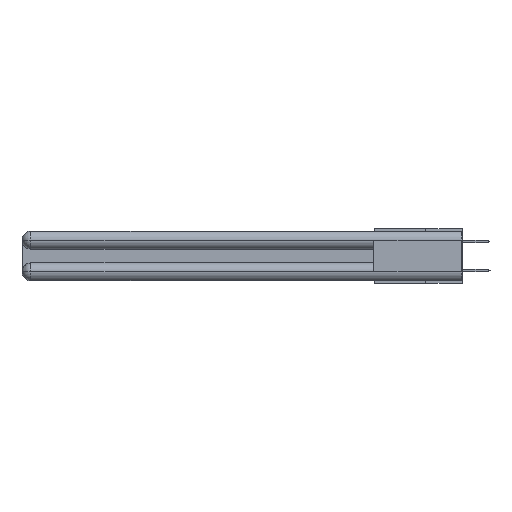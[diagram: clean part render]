
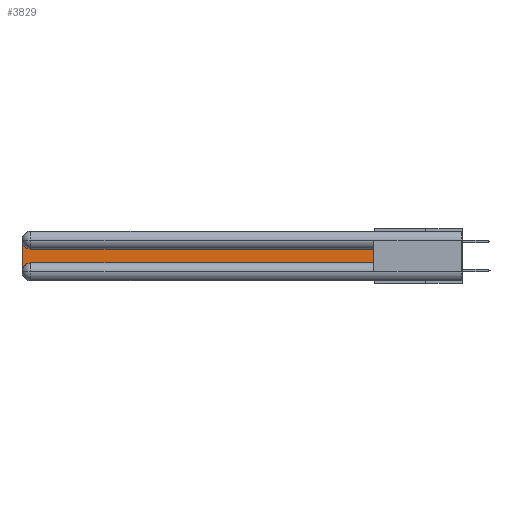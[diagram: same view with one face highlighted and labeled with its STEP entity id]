
A CAD part, left-side view. The second image highlights one B-rep face of the part: STEP entity #3829.
In plain terms, the highlighted planar face has unit normal (-1, 0, 0).
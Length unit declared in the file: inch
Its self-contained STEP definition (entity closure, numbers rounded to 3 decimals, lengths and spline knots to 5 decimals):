
#58 = DIRECTION ( 'NONE',  ( 0., 0., 1. ) ) ;
#1178 = CIRCLE ( 'NONE', #17197, 0.06 ) ;
#1445 = VECTOR ( 'NONE', #58, 39.37008 ) ;
#2576 = VECTOR ( 'NONE', #8021, 39.37008 ) ;
#2670 = CARTESIAN_POINT ( 'NONE',  ( 0.075, 3., -0.0625 ) ) ;
#2958 = PLANE ( 'NONE',  #8251 ) ;
#3028 = EDGE_CURVE ( 'NONE', #10131, #6371, #24535, .T. ) ;
#3141 = DIRECTION ( 'NONE',  ( 1., 0., 0. ) ) ;
#3829 = ADVANCED_FACE ( 'NONE', ( #7758 ), #2958, .F. ) ;
#3873 = CARTESIAN_POINT ( 'NONE',  ( 0.075, 0.6, -0.2175 ) ) ;
#4285 = DIRECTION ( 'NONE',  ( 0., 1., 0. ) ) ;
#4865 = EDGE_CURVE ( 'NONE', #14821, #15504, #6670, .T. ) ;
#5392 = ORIENTED_EDGE ( 'NONE', *, *, #4865, .T. ) ;
#5545 = ORIENTED_EDGE ( 'NONE', *, *, #15381, .T. ) ;
#6146 = CARTESIAN_POINT ( 'NONE',  ( 0.075, 2.94, -0.0625 ) ) ;
#6371 = VERTEX_POINT ( 'NONE', #9166 ) ;
#6670 = LINE ( 'NONE', #3873, #2576 ) ;
#7074 = EDGE_CURVE ( 'NONE', #27422, #10131, #8944, .T. ) ;
#7758 = FACE_OUTER_BOUND ( 'NONE', #18519, .T. ) ;
#7815 = VECTOR ( 'NONE', #28154, 39.37008 ) ;
#7866 = CARTESIAN_POINT ( 'NONE',  ( 0.075, 0.6, -0.2175 ) ) ;
#7909 = EDGE_CURVE ( 'NONE', #27952, #27422, #17935, .T. ) ;
#8021 = DIRECTION ( 'NONE',  ( 0., -1., 0. ) ) ;
#8251 = AXIS2_PLACEMENT_3D ( 'NONE', #16170, #3141, #18395 ) ;
#8944 = CIRCLE ( 'NONE', #21641, 0.06 ) ;
#9101 = CARTESIAN_POINT ( 'NONE',  ( 0.075, 2.94, -0.2775 ) ) ;
#9166 = CARTESIAN_POINT ( 'NONE',  ( 0.075, 3., -0.2775 ) ) ;
#10131 = VERTEX_POINT ( 'NONE', #2670 ) ;
#10805 = CARTESIAN_POINT ( 'NONE',  ( 0.075, 0.6, -0.2175 ) ) ;
#11217 = EDGE_CURVE ( 'NONE', #15504, #27952, #22211, .T. ) ;
#12655 = CARTESIAN_POINT ( 'NONE',  ( 0.075, 2.94, -0.2175 ) ) ;
#14821 = VERTEX_POINT ( 'NONE', #12655 ) ;
#15381 = EDGE_CURVE ( 'NONE', #6371, #14821, #1178, .T. ) ;
#15504 = VERTEX_POINT ( 'NONE', #7866 ) ;
#15704 = ORIENTED_EDGE ( 'NONE', *, *, #3028, .T. ) ;
#16170 = CARTESIAN_POINT ( 'NONE',  ( 0.075, 3., -0.1225 ) ) ;
#17197 = AXIS2_PLACEMENT_3D ( 'NONE', #9101, #25981, #24381 ) ;
#17312 = CARTESIAN_POINT ( 'NONE',  ( 0.075, 0.6, -0.1225 ) ) ;
#17377 = CARTESIAN_POINT ( 'NONE',  ( 0.075, 3., -0.2175 ) ) ;
#17935 = LINE ( 'NONE', #17312, #23753 ) ;
#18395 = DIRECTION ( 'NONE',  ( 0., 0., -1. ) ) ;
#18519 = EDGE_LOOP ( 'NONE', ( #23329, #25066, #15704, #5545, #5392, #22418 ) ) ;
#21641 = AXIS2_PLACEMENT_3D ( 'NONE', #6146, #21686, #23689 ) ;
#21686 = DIRECTION ( 'NONE',  ( 1., 0., 0. ) ) ;
#22211 = LINE ( 'NONE', #10805, #1445 ) ;
#22418 = ORIENTED_EDGE ( 'NONE', *, *, #11217, .T. ) ;
#23329 = ORIENTED_EDGE ( 'NONE', *, *, #7909, .T. ) ;
#23689 = DIRECTION ( 'NONE',  ( 0., 0., -1. ) ) ;
#23753 = VECTOR ( 'NONE', #4285, 39.37008 ) ;
#24381 = DIRECTION ( 'NONE',  ( 0., 0., -1. ) ) ;
#24535 = LINE ( 'NONE', #17377, #7815 ) ;
#25066 = ORIENTED_EDGE ( 'NONE', *, *, #7074, .T. ) ;
#25699 = CARTESIAN_POINT ( 'NONE',  ( 0.075, 2.94, -0.1225 ) ) ;
#25936 = CARTESIAN_POINT ( 'NONE',  ( 0.075, 0.6, -0.1225 ) ) ;
#25981 = DIRECTION ( 'NONE',  ( 1., 0., 0. ) ) ;
#27422 = VERTEX_POINT ( 'NONE', #25699 ) ;
#27952 = VERTEX_POINT ( 'NONE', #25936 ) ;
#28154 = DIRECTION ( 'NONE',  ( 0., 0., -1. ) ) ;
